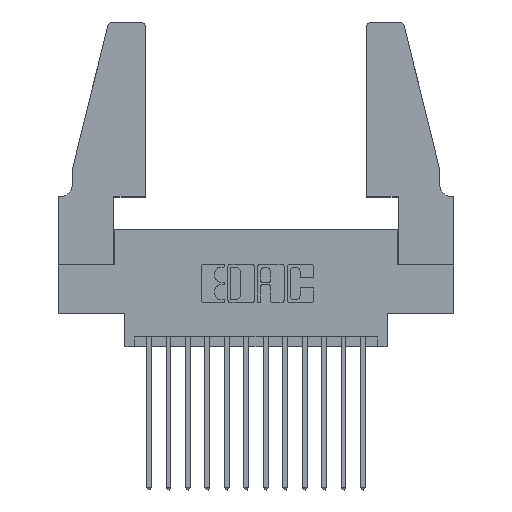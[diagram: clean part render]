
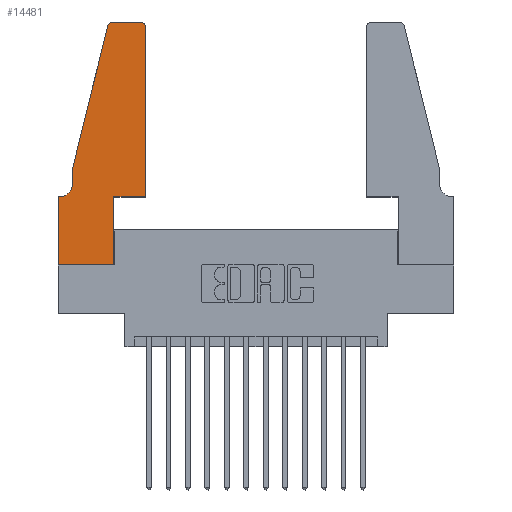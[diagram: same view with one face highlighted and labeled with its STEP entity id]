
A CAD part, top view. The second image highlights one B-rep face of the part: STEP entity #14481.
In plain terms, the highlighted planar face has unit normal (0, 0, 1).
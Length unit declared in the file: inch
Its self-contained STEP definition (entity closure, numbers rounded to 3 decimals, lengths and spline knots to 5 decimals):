
#100 = EDGE_LOOP ( 'NONE', ( #14188, #11348, #5300, #11725, #2771, #12497, #6430, #9626, #10017, #13242, #7175, #7567 ) ) ;
#143 = CARTESIAN_POINT ( 'NONE',  ( 0., 0.35, 0.37 ) ) ;
#258 = DIRECTION ( 'NONE',  ( 0., 1., 0. ) ) ;
#380 = EDGE_CURVE ( 'NONE', #5987, #13754, #533, .T. ) ;
#450 = DIRECTION ( 'NONE',  ( 0., 0., 1. ) ) ;
#533 = LINE ( 'NONE', #6245, #13506 ) ;
#570 = DIRECTION ( 'NONE',  ( 0., 0., 1. ) ) ;
#585 = CARTESIAN_POINT ( 'NONE',  ( 0.4205, 1.22, 0.37 ) ) ;
#969 = DIRECTION ( 'NONE',  ( 0., -1., 0. ) ) ;
#1678 = LINE ( 'NONE', #14869, #4615 ) ;
#1819 = DIRECTION ( 'NONE',  ( 1., 0., 0. ) ) ;
#1828 = VECTOR ( 'NONE', #4861, 39.37008 ) ;
#2202 = DIRECTION ( 'NONE',  ( -0.239, -0.971, 0. ) ) ;
#2280 = EDGE_CURVE ( 'NONE', #12459, #8054, #5875, .T. ) ;
#2551 = CARTESIAN_POINT ( 'NONE',  ( 0.4505, 0.35, 0.37 ) ) ;
#2579 = VECTOR ( 'NONE', #13345, 39.37008 ) ;
#2648 = DIRECTION ( 'NONE',  ( 0., -1., 0. ) ) ;
#2771 = ORIENTED_EDGE ( 'NONE', *, *, #5743, .T. ) ;
#3603 = VERTEX_POINT ( 'NONE', #9557 ) ;
#3744 = VECTOR ( 'NONE', #2648, 39.37008 ) ;
#3842 = DIRECTION ( 'NONE',  ( 1., 0., 0. ) ) ;
#4177 = EDGE_CURVE ( 'NONE', #14106, #10403, #11143, .T. ) ;
#4367 = VECTOR ( 'NONE', #2202, 39.37008 ) ;
#4424 = EDGE_CURVE ( 'NONE', #13754, #12459, #13804, .T. ) ;
#4463 = CARTESIAN_POINT ( 'NONE',  ( 0.2865, 0.35, 0.37 ) ) ;
#4570 = CARTESIAN_POINT ( 'NONE',  ( 0.4205, 1.25, 0.37 ) ) ;
#4615 = VECTOR ( 'NONE', #258, 39.37008 ) ;
#4657 = LINE ( 'NONE', #14371, #7472 ) ;
#4861 = DIRECTION ( 'NONE',  ( -1., 0., 0. ) ) ;
#4864 = AXIS2_PLACEMENT_3D ( 'NONE', #6718, #570, #9147 ) ;
#4886 = VERTEX_POINT ( 'NONE', #5636 ) ;
#5300 = ORIENTED_EDGE ( 'NONE', *, *, #4177, .T. ) ;
#5636 = CARTESIAN_POINT ( 'NONE',  ( 0.4505, 0.35, 0.37 ) ) ;
#5743 = EDGE_CURVE ( 'NONE', #14280, #5987, #7298, .T. ) ;
#5875 = LINE ( 'NONE', #10911, #2579 ) ;
#5987 = VERTEX_POINT ( 'NONE', #7871 ) ;
#6237 = CARTESIAN_POINT ( 'NONE',  ( 0.0055, 0.42, 0.37 ) ) ;
#6245 = CARTESIAN_POINT ( 'NONE',  ( 0.0755, 0.35, 0.37 ) ) ;
#6430 = ORIENTED_EDGE ( 'NONE', *, *, #4424, .T. ) ;
#6718 = CARTESIAN_POINT ( 'NONE',  ( 0., 0.35, 0.37 ) ) ;
#6969 = CARTESIAN_POINT ( 'NONE',  ( 0.2865, 0., 0.37 ) ) ;
#7175 = ORIENTED_EDGE ( 'NONE', *, *, #9119, .T. ) ;
#7188 = CARTESIAN_POINT ( 'NONE',  ( 0.25487, 1.22718, 0.37 ) ) ;
#7298 = CIRCLE ( 'NONE', #7388, 0.07 ) ;
#7388 = AXIS2_PLACEMENT_3D ( 'NONE', #6237, #14705, #7448 ) ;
#7416 = VERTEX_POINT ( 'NONE', #4463 ) ;
#7448 = DIRECTION ( 'NONE',  ( -1., 0., 0. ) ) ;
#7472 = VECTOR ( 'NONE', #969, 39.37008 ) ;
#7567 = ORIENTED_EDGE ( 'NONE', *, *, #15754, .T. ) ;
#7673 = FACE_OUTER_BOUND ( 'NONE', #100, .T. ) ;
#7800 = CARTESIAN_POINT ( 'NONE',  ( 0.284, 1.22, 0.37 ) ) ;
#7824 = VERTEX_POINT ( 'NONE', #8932 ) ;
#7871 = CARTESIAN_POINT ( 'NONE',  ( 0.0055, 0.35, 0.37 ) ) ;
#7925 = PLANE ( 'NONE',  #4864 ) ;
#7993 = CARTESIAN_POINT ( 'NONE',  ( 0., 0., 0.37 ) ) ;
#8054 = VERTEX_POINT ( 'NONE', #6969 ) ;
#8311 = CARTESIAN_POINT ( 'NONE',  ( 0.0755, 0.5, 0.37 ) ) ;
#8496 = AXIS2_PLACEMENT_3D ( 'NONE', #585, #9164, #1819 ) ;
#8932 = CARTESIAN_POINT ( 'NONE',  ( 0.284, 1.25, 0.37 ) ) ;
#9018 = DIRECTION ( 'NONE',  ( 1., 0., 0. ) ) ;
#9119 = EDGE_CURVE ( 'NONE', #4886, #3603, #1678, .T. ) ;
#9130 = LINE ( 'NONE', #2551, #15187 ) ;
#9147 = DIRECTION ( 'NONE',  ( 1., 0., 0. ) ) ;
#9164 = DIRECTION ( 'NONE',  ( 0., 0., 1. ) ) ;
#9557 = CARTESIAN_POINT ( 'NONE',  ( 0.4505, 1.22, 0.37 ) ) ;
#9626 = ORIENTED_EDGE ( 'NONE', *, *, #2280, .T. ) ;
#9666 = EDGE_CURVE ( 'NONE', #7416, #4886, #9130, .T. ) ;
#9982 = CARTESIAN_POINT ( 'NONE',  ( 0.0755, 0.42, 0.37 ) ) ;
#10017 = ORIENTED_EDGE ( 'NONE', *, *, #10419, .T. ) ;
#10106 = EDGE_CURVE ( 'NONE', #12518, #7824, #11574, .T. ) ;
#10244 = VECTOR ( 'NONE', #10245, 39.37008 ) ;
#10245 = DIRECTION ( 'NONE',  ( 0., 1., 0. ) ) ;
#10403 = VERTEX_POINT ( 'NONE', #11354 ) ;
#10411 = EDGE_CURVE ( 'NONE', #7824, #14106, #14975, .T. ) ;
#10419 = EDGE_CURVE ( 'NONE', #8054, #7416, #13455, .T. ) ;
#10911 = CARTESIAN_POINT ( 'NONE',  ( 0., 0., 0.37 ) ) ;
#11143 = LINE ( 'NONE', #8311, #4367 ) ;
#11181 = CARTESIAN_POINT ( 'NONE',  ( 0., 0., 0.37 ) ) ;
#11348 = ORIENTED_EDGE ( 'NONE', *, *, #10411, .T. ) ;
#11354 = CARTESIAN_POINT ( 'NONE',  ( 0.0755, 0.5, 0.37 ) ) ;
#11574 = LINE ( 'NONE', #13308, #1828 ) ;
#11725 = ORIENTED_EDGE ( 'NONE', *, *, #14726, .T. ) ;
#11975 = CIRCLE ( 'NONE', #8496, 0.03 ) ;
#12459 = VERTEX_POINT ( 'NONE', #7993 ) ;
#12497 = ORIENTED_EDGE ( 'NONE', *, *, #380, .T. ) ;
#12518 = VERTEX_POINT ( 'NONE', #4570 ) ;
#13110 = AXIS2_PLACEMENT_3D ( 'NONE', #7800, #450, #9018 ) ;
#13242 = ORIENTED_EDGE ( 'NONE', *, *, #9666, .T. ) ;
#13308 = CARTESIAN_POINT ( 'NONE',  ( 0.2605, 1.25, 0.37 ) ) ;
#13326 = DIRECTION ( 'NONE',  ( -1., 0., 0. ) ) ;
#13345 = DIRECTION ( 'NONE',  ( 1., 0., 0. ) ) ;
#13455 = LINE ( 'NONE', #15002, #10244 ) ;
#13506 = VECTOR ( 'NONE', #13326, 39.37008 ) ;
#13754 = VERTEX_POINT ( 'NONE', #143 ) ;
#13804 = LINE ( 'NONE', #11181, #3744 ) ;
#14106 = VERTEX_POINT ( 'NONE', #7188 ) ;
#14188 = ORIENTED_EDGE ( 'NONE', *, *, #10106, .T. ) ;
#14280 = VERTEX_POINT ( 'NONE', #9982 ) ;
#14371 = CARTESIAN_POINT ( 'NONE',  ( 0.0755, 0.5, 0.37 ) ) ;
#14481 = ADVANCED_FACE ( 'NONE', ( #7673 ), #7925, .T. ) ;
#14705 = DIRECTION ( 'NONE',  ( 0., 0., -1. ) ) ;
#14726 = EDGE_CURVE ( 'NONE', #10403, #14280, #4657, .T. ) ;
#14869 = CARTESIAN_POINT ( 'NONE',  ( 0.4505, 0.35, 0.37 ) ) ;
#14975 = CIRCLE ( 'NONE', #13110, 0.03 ) ;
#15002 = CARTESIAN_POINT ( 'NONE',  ( 0.2865, 0.35, 0.37 ) ) ;
#15187 = VECTOR ( 'NONE', #3842, 39.37008 ) ;
#15754 = EDGE_CURVE ( 'NONE', #3603, #12518, #11975, .T. ) ;
